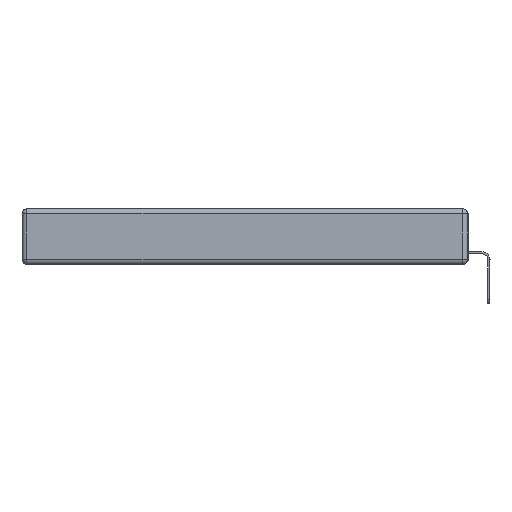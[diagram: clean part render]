
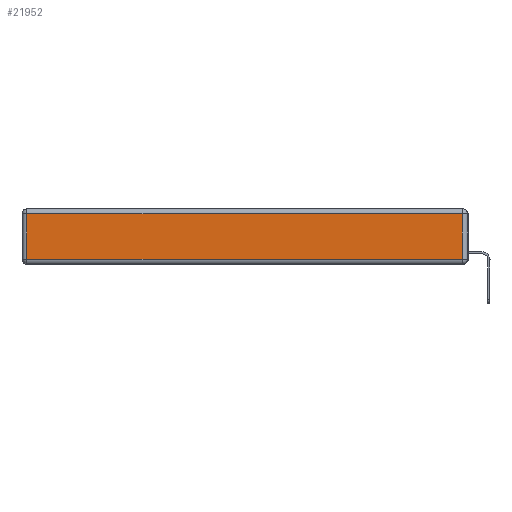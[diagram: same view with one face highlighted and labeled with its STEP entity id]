
A CAD part, left-side view. The second image highlights one B-rep face of the part: STEP entity #21952.
In plain terms, the highlighted planar face has unit normal (-1, 0, 0).
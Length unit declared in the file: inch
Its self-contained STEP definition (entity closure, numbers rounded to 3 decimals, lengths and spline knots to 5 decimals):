
#194 = CARTESIAN_POINT ( 'NONE',  ( 0., 0.03, -0.03 ) ) ;
#504 = AXIS2_PLACEMENT_3D ( 'NONE', #20144, #7816, #24249 ) ;
#542 = CARTESIAN_POINT ( 'NONE',  ( 0., 0., -0.313 ) ) ;
#3572 = VERTEX_POINT ( 'NONE', #8421 ) ;
#4326 = CARTESIAN_POINT ( 'NONE',  ( 0., 0.03, -0.343 ) ) ;
#4641 = DIRECTION ( 'NONE',  ( 0., -1., 0. ) ) ;
#5291 = ORIENTED_EDGE ( 'NONE', *, *, #20320, .T. ) ;
#5336 = CARTESIAN_POINT ( 'NONE',  ( 0., 0.03, -0.313 ) ) ;
#5784 = PLANE ( 'NONE',  #504 ) ;
#6350 = VECTOR ( 'NONE', #14692, 39.37008 ) ;
#7209 = DIRECTION ( 'NONE',  ( 0., 0., -1. ) ) ;
#7816 = DIRECTION ( 'NONE',  ( -1., 0., 0. ) ) ;
#8188 = LINE ( 'NONE', #542, #18697 ) ;
#8421 = CARTESIAN_POINT ( 'NONE',  ( 0., 2.72, -0.03 ) ) ;
#8516 = CARTESIAN_POINT ( 'NONE',  ( 0., 2.75, -0.03 ) ) ;
#8570 = VERTEX_POINT ( 'NONE', #13529 ) ;
#10854 = FACE_OUTER_BOUND ( 'NONE', #25877, .T. ) ;
#10918 = EDGE_CURVE ( 'NONE', #18636, #16124, #16180, .T. ) ;
#12684 = LINE ( 'NONE', #19349, #20626 ) ;
#13529 = CARTESIAN_POINT ( 'NONE',  ( 0., 2.72, -0.313 ) ) ;
#14692 = DIRECTION ( 'NONE',  ( 0., 1., 0. ) ) ;
#15061 = ORIENTED_EDGE ( 'NONE', *, *, #20613, .T. ) ;
#16124 = VERTEX_POINT ( 'NONE', #194 ) ;
#16134 = LINE ( 'NONE', #8516, #6350 ) ;
#16180 = LINE ( 'NONE', #4326, #20963 ) ;
#16757 = ORIENTED_EDGE ( 'NONE', *, *, #10918, .T. ) ;
#18244 = DIRECTION ( 'NONE',  ( 0., 0., 1. ) ) ;
#18636 = VERTEX_POINT ( 'NONE', #5336 ) ;
#18697 = VECTOR ( 'NONE', #4641, 39.37008 ) ;
#19349 = CARTESIAN_POINT ( 'NONE',  ( 0., 2.72, -0.343 ) ) ;
#20144 = CARTESIAN_POINT ( 'NONE',  ( 0., 0., -0.343 ) ) ;
#20320 = EDGE_CURVE ( 'NONE', #3572, #8570, #12684, .T. ) ;
#20613 = EDGE_CURVE ( 'NONE', #16124, #3572, #16134, .T. ) ;
#20626 = VECTOR ( 'NONE', #7209, 39.37008 ) ;
#20963 = VECTOR ( 'NONE', #18244, 39.37008 ) ;
#21769 = ORIENTED_EDGE ( 'NONE', *, *, #25064, .T. ) ;
#21952 = ADVANCED_FACE ( 'NONE', ( #10854 ), #5784, .T. ) ;
#24249 = DIRECTION ( 'NONE',  ( 0., 0., 1. ) ) ;
#25064 = EDGE_CURVE ( 'NONE', #8570, #18636, #8188, .T. ) ;
#25877 = EDGE_LOOP ( 'NONE', ( #21769, #16757, #15061, #5291 ) ) ;
